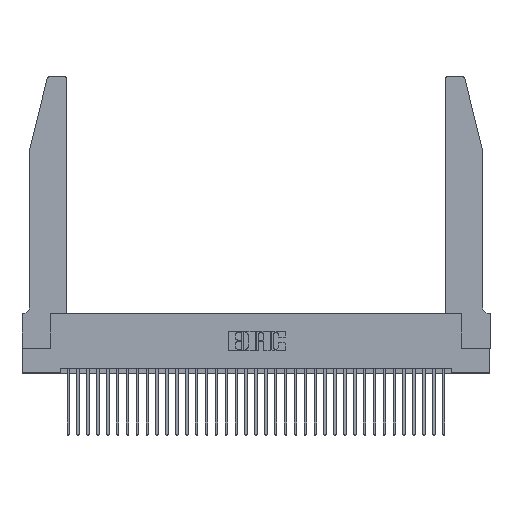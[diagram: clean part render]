
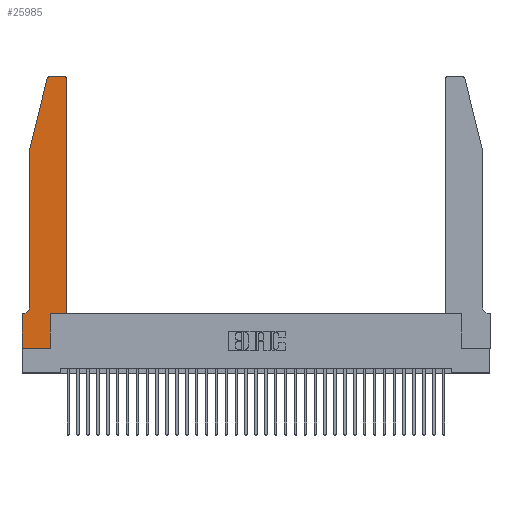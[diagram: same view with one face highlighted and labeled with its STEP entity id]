
A CAD part, top view. The second image highlights one B-rep face of the part: STEP entity #25985.
In plain terms, the highlighted planar face has unit normal (0, 0, 1).
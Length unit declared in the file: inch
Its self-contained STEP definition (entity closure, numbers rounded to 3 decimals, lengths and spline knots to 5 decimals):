
#149 = CARTESIAN_POINT ( 'NONE',  ( 0.0755, 2., 0.37 ) ) ;
#839 = ORIENTED_EDGE ( 'NONE', *, *, #29169, .T. ) ;
#1187 = EDGE_CURVE ( 'NONE', #23807, #17869, #17261, .T. ) ;
#1841 = VECTOR ( 'NONE', #23195, 39.37008 ) ;
#2741 = CARTESIAN_POINT ( 'NONE',  ( 0., 0., 0.37 ) ) ;
#3551 = CARTESIAN_POINT ( 'NONE',  ( 0.4505, 0.35, 0.37 ) ) ;
#4756 = VECTOR ( 'NONE', #17978, 39.37008 ) ;
#4916 = LINE ( 'NONE', #149, #11362 ) ;
#5037 = EDGE_CURVE ( 'NONE', #20416, #20159, #32202, .T. ) ;
#5156 = CARTESIAN_POINT ( 'NONE',  ( 0.2865, 0.35, 0.37 ) ) ;
#5190 = CARTESIAN_POINT ( 'NONE',  ( 0.0755, 2., 0.37 ) ) ;
#5353 = LINE ( 'NONE', #9535, #30769 ) ;
#5490 = AXIS2_PLACEMENT_3D ( 'NONE', #26443, #35362, #18313 ) ;
#5605 = PLANE ( 'NONE',  #18107 ) ;
#5714 = CARTESIAN_POINT ( 'NONE',  ( 0.25487, 2.72718, 0.37 ) ) ;
#5859 = ORIENTED_EDGE ( 'NONE', *, *, #1187, .T. ) ;
#6218 = EDGE_CURVE ( 'NONE', #17869, #23085, #14622, .T. ) ;
#6871 = ORIENTED_EDGE ( 'NONE', *, *, #22976, .T. ) ;
#7022 = EDGE_CURVE ( 'NONE', #29002, #21134, #5353, .T. ) ;
#9535 = CARTESIAN_POINT ( 'NONE',  ( 0.2865, 0.35, 0.37 ) ) ;
#9748 = VERTEX_POINT ( 'NONE', #32388 ) ;
#11102 = DIRECTION ( 'NONE',  ( 1., 0., 0. ) ) ;
#11362 = VECTOR ( 'NONE', #33152, 39.37008 ) ;
#11390 = ORIENTED_EDGE ( 'NONE', *, *, #18691, .T. ) ;
#11417 = DIRECTION ( 'NONE',  ( 0., 1., 0. ) ) ;
#11455 = EDGE_CURVE ( 'NONE', #20159, #27094, #14484, .T. ) ;
#12531 = CARTESIAN_POINT ( 'NONE',  ( 0.2865, 0., 0.37 ) ) ;
#12679 = LINE ( 'NONE', #25707, #1841 ) ;
#14023 = DIRECTION ( 'NONE',  ( 1., 0., 0. ) ) ;
#14056 = DIRECTION ( 'NONE',  ( 1., 0., 0. ) ) ;
#14484 = CIRCLE ( 'NONE', #16920, 0.03 ) ;
#14622 = LINE ( 'NONE', #20497, #4756 ) ;
#15232 = CARTESIAN_POINT ( 'NONE',  ( 0., 0., 0.37 ) ) ;
#15464 = VECTOR ( 'NONE', #28312, 39.37008 ) ;
#15471 = ORIENTED_EDGE ( 'NONE', *, *, #35250, .T. ) ;
#15967 = EDGE_CURVE ( 'NONE', #21134, #20416, #30973, .T. ) ;
#16050 = CARTESIAN_POINT ( 'NONE',  ( 0.4205, 2.72, 0.37 ) ) ;
#16282 = VECTOR ( 'NONE', #27065, 39.37008 ) ;
#16920 = AXIS2_PLACEMENT_3D ( 'NONE', #16050, #32843, #11102 ) ;
#17033 = EDGE_CURVE ( 'NONE', #30089, #9748, #33549, .T. ) ;
#17261 = CIRCLE ( 'NONE', #25422, 0.07 ) ;
#17363 = DIRECTION ( 'NONE',  ( 0., 0., -1. ) ) ;
#17869 = VERTEX_POINT ( 'NONE', #24289 ) ;
#17944 = ORIENTED_EDGE ( 'NONE', *, *, #5037, .T. ) ;
#17978 = DIRECTION ( 'NONE',  ( -1., 0., 0. ) ) ;
#18107 = AXIS2_PLACEMENT_3D ( 'NONE', #27613, #24753, #14023 ) ;
#18313 = DIRECTION ( 'NONE',  ( 1., 0., 0. ) ) ;
#18366 = CARTESIAN_POINT ( 'NONE',  ( 0.4505, 0.35, 0.37 ) ) ;
#18408 = VECTOR ( 'NONE', #14056, 39.37008 ) ;
#18584 = CARTESIAN_POINT ( 'NONE',  ( 0.284, 2.75, 0.37 ) ) ;
#18691 = EDGE_CURVE ( 'NONE', #31121, #30089, #35187, .T. ) ;
#19292 = VECTOR ( 'NONE', #22192, 39.37008 ) ;
#19646 = LINE ( 'NONE', #2741, #18408 ) ;
#20159 = VERTEX_POINT ( 'NONE', #22956 ) ;
#20416 = VERTEX_POINT ( 'NONE', #18366 ) ;
#20497 = CARTESIAN_POINT ( 'NONE',  ( 0.0755, 0.35, 0.37 ) ) ;
#20920 = ORIENTED_EDGE ( 'NONE', *, *, #17033, .T. ) ;
#21134 = VERTEX_POINT ( 'NONE', #5156 ) ;
#22192 = DIRECTION ( 'NONE',  ( -1., 0., 0. ) ) ;
#22779 = ORIENTED_EDGE ( 'NONE', *, *, #15967, .T. ) ;
#22956 = CARTESIAN_POINT ( 'NONE',  ( 0.4505, 2.72, 0.37 ) ) ;
#22976 = EDGE_CURVE ( 'NONE', #27094, #31121, #31316, .T. ) ;
#23085 = VERTEX_POINT ( 'NONE', #23415 ) ;
#23195 = DIRECTION ( 'NONE',  ( 0., -1., 0. ) ) ;
#23415 = CARTESIAN_POINT ( 'NONE',  ( 0., 0.35, 0.37 ) ) ;
#23469 = CARTESIAN_POINT ( 'NONE',  ( 0.4205, 2.75, 0.37 ) ) ;
#23807 = VERTEX_POINT ( 'NONE', #35351 ) ;
#24194 = EDGE_CURVE ( 'NONE', #31668, #29002, #19646, .T. ) ;
#24289 = CARTESIAN_POINT ( 'NONE',  ( 0.0055, 0.35, 0.37 ) ) ;
#24753 = DIRECTION ( 'NONE',  ( 0., 0., 1. ) ) ;
#24819 = ORIENTED_EDGE ( 'NONE', *, *, #24194, .T. ) ;
#25422 = AXIS2_PLACEMENT_3D ( 'NONE', #27942, #17363, #33794 ) ;
#25707 = CARTESIAN_POINT ( 'NONE',  ( 0., 0., 0.37 ) ) ;
#25842 = ORIENTED_EDGE ( 'NONE', *, *, #7022, .T. ) ;
#25985 = ADVANCED_FACE ( 'NONE', ( #26396 ), #5605, .T. ) ;
#26396 = FACE_OUTER_BOUND ( 'NONE', #26489, .T. ) ;
#26443 = CARTESIAN_POINT ( 'NONE',  ( 0.284, 2.72, 0.37 ) ) ;
#26489 = EDGE_LOOP ( 'NONE', ( #6871, #11390, #20920, #839, #5859, #28216, #15471, #24819, #25842, #22779, #17944, #35508 ) ) ;
#26996 = DIRECTION ( 'NONE',  ( 0., 1., 0. ) ) ;
#27065 = DIRECTION ( 'NONE',  ( -0.239, -0.971, 0. ) ) ;
#27094 = VERTEX_POINT ( 'NONE', #23469 ) ;
#27613 = CARTESIAN_POINT ( 'NONE',  ( 0., 0.35, 0.37 ) ) ;
#27942 = CARTESIAN_POINT ( 'NONE',  ( 0.0055, 0.42, 0.37 ) ) ;
#28216 = ORIENTED_EDGE ( 'NONE', *, *, #6218, .T. ) ;
#28312 = DIRECTION ( 'NONE',  ( 1., 0., 0. ) ) ;
#29002 = VERTEX_POINT ( 'NONE', #12531 ) ;
#29169 = EDGE_CURVE ( 'NONE', #9748, #23807, #4916, .T. ) ;
#30089 = VERTEX_POINT ( 'NONE', #5714 ) ;
#30769 = VECTOR ( 'NONE', #11417, 39.37008 ) ;
#30973 = LINE ( 'NONE', #3551, #15464 ) ;
#31121 = VERTEX_POINT ( 'NONE', #18584 ) ;
#31316 = LINE ( 'NONE', #33718, #19292 ) ;
#31668 = VERTEX_POINT ( 'NONE', #15232 ) ;
#32202 = LINE ( 'NONE', #35431, #35271 ) ;
#32388 = CARTESIAN_POINT ( 'NONE',  ( 0.0755, 2., 0.37 ) ) ;
#32843 = DIRECTION ( 'NONE',  ( 0., 0., 1. ) ) ;
#33152 = DIRECTION ( 'NONE',  ( 0., -1., 0. ) ) ;
#33549 = LINE ( 'NONE', #5190, #16282 ) ;
#33718 = CARTESIAN_POINT ( 'NONE',  ( 0.2605, 2.75, 0.37 ) ) ;
#33794 = DIRECTION ( 'NONE',  ( -1., 0., 0. ) ) ;
#35187 = CIRCLE ( 'NONE', #5490, 0.03 ) ;
#35250 = EDGE_CURVE ( 'NONE', #23085, #31668, #12679, .T. ) ;
#35271 = VECTOR ( 'NONE', #26996, 39.37008 ) ;
#35351 = CARTESIAN_POINT ( 'NONE',  ( 0.0755, 0.42, 0.37 ) ) ;
#35362 = DIRECTION ( 'NONE',  ( 0., 0., 1. ) ) ;
#35431 = CARTESIAN_POINT ( 'NONE',  ( 0.4505, 0.35, 0.37 ) ) ;
#35508 = ORIENTED_EDGE ( 'NONE', *, *, #11455, .T. ) ;
